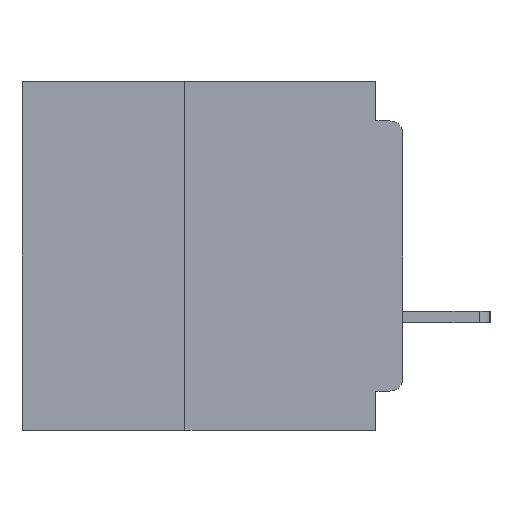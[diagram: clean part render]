
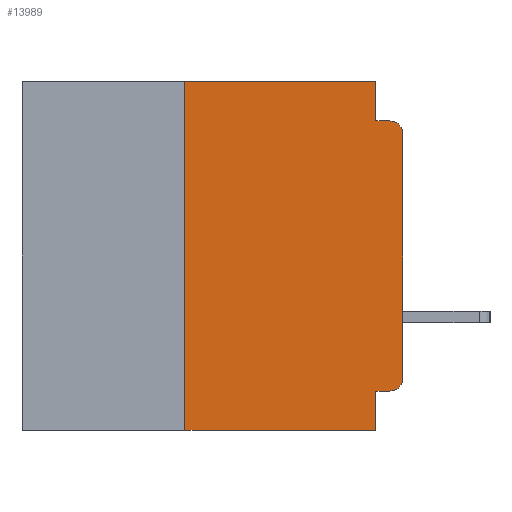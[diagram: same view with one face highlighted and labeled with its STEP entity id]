
A CAD part, left-side view. The second image highlights one B-rep face of the part: STEP entity #13989.
In plain terms, the highlighted planar face has unit normal (-1, 0, 0).
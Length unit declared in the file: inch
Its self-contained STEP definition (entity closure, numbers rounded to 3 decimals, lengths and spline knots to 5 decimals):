
#873 = CARTESIAN_POINT ( 'NONE',  ( 0., 0., -0.045 ) ) ;
#1386 = EDGE_CURVE ( 'NONE', #28791, #12751, #46641, .T. ) ;
#2573 = VERTEX_POINT ( 'NONE', #15252 ) ;
#2790 = ORIENTED_EDGE ( 'NONE', *, *, #47308, .F. ) ;
#3839 = CARTESIAN_POINT ( 'NONE',  ( 0., 0.015, -0.06 ) ) ;
#4741 = ORIENTED_EDGE ( 'NONE', *, *, #37132, .T. ) ;
#5556 = ORIENTED_EDGE ( 'NONE', *, *, #42618, .F. ) ;
#6519 = CARTESIAN_POINT ( 'NONE',  ( 0., 0.25, 0. ) ) ;
#6548 = VECTOR ( 'NONE', #49206, 39.37008 ) ;
#6567 = DIRECTION ( 'NONE',  ( 0., 0., 1. ) ) ;
#6678 = CARTESIAN_POINT ( 'NONE',  ( 0., 0.031, 0. ) ) ;
#7852 = DIRECTION ( 'NONE',  ( 0., 0., -1. ) ) ;
#10367 = LINE ( 'NONE', #41826, #19455 ) ;
#11034 = EDGE_CURVE ( 'NONE', #13341, #44605, #22318, .T. ) ;
#11295 = AXIS2_PLACEMENT_3D ( 'NONE', #36083, #47709, #24384 ) ;
#11348 = CARTESIAN_POINT ( 'NONE',  ( 0., 0.437, -0.4 ) ) ;
#11997 = ORIENTED_EDGE ( 'NONE', *, *, #47368, .F. ) ;
#12005 = VECTOR ( 'NONE', #15286, 39.37008 ) ;
#12359 = CARTESIAN_POINT ( 'NONE',  ( 0., 0.25, -0.4 ) ) ;
#12751 = VERTEX_POINT ( 'NONE', #20709 ) ;
#12953 = VECTOR ( 'NONE', #44434, 39.37008 ) ;
#13341 = VERTEX_POINT ( 'NONE', #12359 ) ;
#13987 = CARTESIAN_POINT ( 'NONE',  ( 0., 0., -0.355 ) ) ;
#13989 = ADVANCED_FACE ( 'NONE', ( #26424 ), #20407, .F. ) ;
#14736 = DIRECTION ( 'NONE',  ( -1., 0., 0. ) ) ;
#15252 = CARTESIAN_POINT ( 'NONE',  ( 0., 0.031, -0.355 ) ) ;
#15286 = DIRECTION ( 'NONE',  ( 0., -1., 0. ) ) ;
#15747 = LINE ( 'NONE', #41850, #16936 ) ;
#16936 = VECTOR ( 'NONE', #30265, 39.37008 ) ;
#17112 = CARTESIAN_POINT ( 'NONE',  ( 0., 0.437, 0. ) ) ;
#18135 = VERTEX_POINT ( 'NONE', #19313 ) ;
#18230 = EDGE_LOOP ( 'NONE', ( #35805, #29093, #48739, #31930, #5556, #30133, #45557, #11997, #2790, #4741 ) ) ;
#19313 = CARTESIAN_POINT ( 'NONE',  ( 0., 0.031, -0.045 ) ) ;
#19455 = VECTOR ( 'NONE', #6567, 39.37008 ) ;
#20407 = PLANE ( 'NONE',  #11295 ) ;
#20603 = DIRECTION ( 'NONE',  ( 0., -1., 0. ) ) ;
#20709 = CARTESIAN_POINT ( 'NONE',  ( 0., 0., -0.06 ) ) ;
#22318 = LINE ( 'NONE', #11348, #12005 ) ;
#24340 = AXIS2_PLACEMENT_3D ( 'NONE', #3839, #31315, #7852 ) ;
#24384 = DIRECTION ( 'NONE',  ( 0., 0., -1. ) ) ;
#25928 = VECTOR ( 'NONE', #42542, 39.37008 ) ;
#26239 = CARTESIAN_POINT ( 'NONE',  ( 0., 0.031, -0.4 ) ) ;
#26424 = FACE_OUTER_BOUND ( 'NONE', #18230, .T. ) ;
#26964 = LINE ( 'NONE', #6678, #37384 ) ;
#27395 = LINE ( 'NONE', #13987, #6548 ) ;
#28473 = EDGE_CURVE ( 'NONE', #37847, #18135, #26964, .T. ) ;
#28791 = VERTEX_POINT ( 'NONE', #31851 ) ;
#29093 = ORIENTED_EDGE ( 'NONE', *, *, #38833, .T. ) ;
#30133 = ORIENTED_EDGE ( 'NONE', *, *, #44595, .F. ) ;
#30265 = DIRECTION ( 'NONE',  ( 0., 0., -1. ) ) ;
#31315 = DIRECTION ( 'NONE',  ( -1., 0., 0. ) ) ;
#31851 = CARTESIAN_POINT ( 'NONE',  ( 0., 0., -0.34 ) ) ;
#31930 = ORIENTED_EDGE ( 'NONE', *, *, #28473, .F. ) ;
#33793 = LINE ( 'NONE', #17112, #12953 ) ;
#34588 = VECTOR ( 'NONE', #20603, 39.37008 ) ;
#35805 = ORIENTED_EDGE ( 'NONE', *, *, #1386, .T. ) ;
#36083 = CARTESIAN_POINT ( 'NONE',  ( 0., 0.437, 0. ) ) ;
#37132 = EDGE_CURVE ( 'NONE', #39195, #28791, #42319, .T. ) ;
#37384 = VECTOR ( 'NONE', #38032, 39.37008 ) ;
#37847 = VERTEX_POINT ( 'NONE', #46708 ) ;
#38032 = DIRECTION ( 'NONE',  ( 0., 0., -1. ) ) ;
#38134 = AXIS2_PLACEMENT_3D ( 'NONE', #38199, #14736, #42092 ) ;
#38199 = CARTESIAN_POINT ( 'NONE',  ( 0., 0.015, -0.34 ) ) ;
#38833 = EDGE_CURVE ( 'NONE', #12751, #50312, #47592, .T. ) ;
#39195 = VERTEX_POINT ( 'NONE', #41328 ) ;
#39891 = VERTEX_POINT ( 'NONE', #6519 ) ;
#41328 = CARTESIAN_POINT ( 'NONE',  ( 0., 0.015, -0.355 ) ) ;
#41826 = CARTESIAN_POINT ( 'NONE',  ( 0., 0.25, -0.4 ) ) ;
#41850 = CARTESIAN_POINT ( 'NONE',  ( 0., 0.031, -0.4 ) ) ;
#42092 = DIRECTION ( 'NONE',  ( 0., 0., -1. ) ) ;
#42319 = CIRCLE ( 'NONE', #38134, 0.015 ) ;
#42369 = CARTESIAN_POINT ( 'NONE',  ( 0., 0., 0. ) ) ;
#42542 = DIRECTION ( 'NONE',  ( 0., 0., 1. ) ) ;
#42618 = EDGE_CURVE ( 'NONE', #39891, #37847, #33793, .T. ) ;
#44434 = DIRECTION ( 'NONE',  ( 0., -1., 0. ) ) ;
#44595 = EDGE_CURVE ( 'NONE', #13341, #39891, #10367, .T. ) ;
#44605 = VERTEX_POINT ( 'NONE', #26239 ) ;
#44877 = LINE ( 'NONE', #873, #34588 ) ;
#45557 = ORIENTED_EDGE ( 'NONE', *, *, #11034, .T. ) ;
#46641 = LINE ( 'NONE', #42369, #25928 ) ;
#46708 = CARTESIAN_POINT ( 'NONE',  ( 0., 0.031, 0. ) ) ;
#47308 = EDGE_CURVE ( 'NONE', #39195, #2573, #27395, .T. ) ;
#47368 = EDGE_CURVE ( 'NONE', #2573, #44605, #15747, .T. ) ;
#47592 = CIRCLE ( 'NONE', #24340, 0.015 ) ;
#47709 = DIRECTION ( 'NONE',  ( 1., 0., 0. ) ) ;
#48739 = ORIENTED_EDGE ( 'NONE', *, *, #48898, .F. ) ;
#48898 = EDGE_CURVE ( 'NONE', #18135, #50312, #44877, .T. ) ;
#49206 = DIRECTION ( 'NONE',  ( 0., 1., 0. ) ) ;
#50082 = CARTESIAN_POINT ( 'NONE',  ( 0., 0.015, -0.045 ) ) ;
#50312 = VERTEX_POINT ( 'NONE', #50082 ) ;
